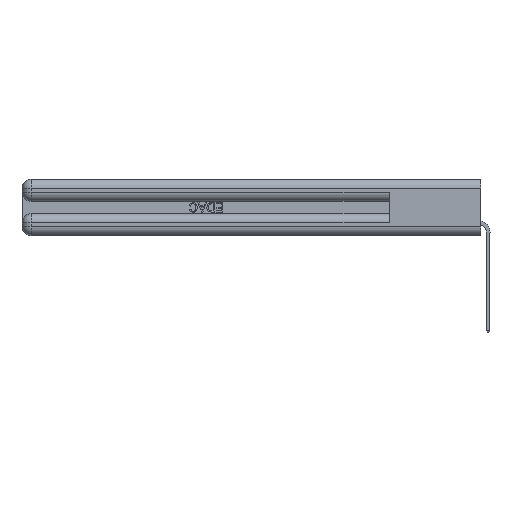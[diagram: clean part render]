
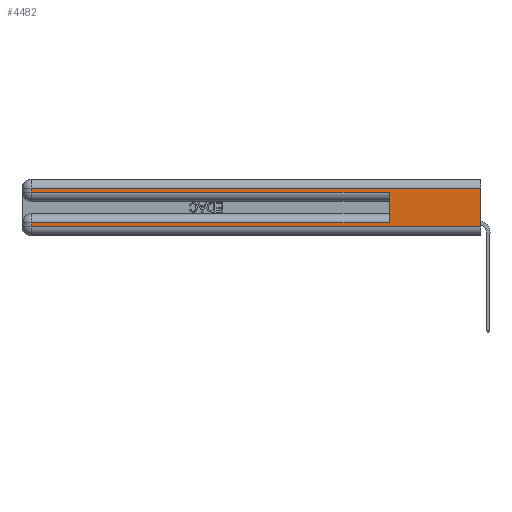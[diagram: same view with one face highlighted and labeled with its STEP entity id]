
A CAD part, left-side view. The second image highlights one B-rep face of the part: STEP entity #4482.
In plain terms, the highlighted planar face has unit normal (-1, 0, 0).
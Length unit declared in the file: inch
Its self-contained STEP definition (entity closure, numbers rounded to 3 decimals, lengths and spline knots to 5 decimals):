
#642 = EDGE_CURVE ( 'NONE', #20522, #5445, #36103, .T. ) ;
#1931 = FACE_OUTER_BOUND ( 'NONE', #25364, .T. ) ;
#2450 = EDGE_CURVE ( 'NONE', #24085, #14892, #4341, .T. ) ;
#4311 = VECTOR ( 'NONE', #20294, 39.37008 ) ;
#4341 = LINE ( 'NONE', #31366, #31011 ) ;
#4423 = ORIENTED_EDGE ( 'NONE', *, *, #25893, .F. ) ;
#4482 = ADVANCED_FACE ( 'NONE', ( #1931 ), #22855, .F. ) ;
#5445 = VERTEX_POINT ( 'NONE', #17617 ) ;
#5885 = DIRECTION ( 'NONE',  ( 1., 0., 0. ) ) ;
#6521 = LINE ( 'NONE', #22173, #24303 ) ;
#6970 = CARTESIAN_POINT ( 'NONE',  ( 0., 2.94, 0.06 ) ) ;
#8982 = ORIENTED_EDGE ( 'NONE', *, *, #10258, .T. ) ;
#9415 = VERTEX_POINT ( 'NONE', #13876 ) ;
#10258 = EDGE_CURVE ( 'NONE', #14892, #24863, #6521, .T. ) ;
#10935 = ORIENTED_EDGE ( 'NONE', *, *, #14495, .T. ) ;
#12194 = VERTEX_POINT ( 'NONE', #35616 ) ;
#13784 = VECTOR ( 'NONE', #21366, 39.37008 ) ;
#13876 = CARTESIAN_POINT ( 'NONE',  ( 0., 2.94, 0.285 ) ) ;
#14004 = CARTESIAN_POINT ( 'NONE',  ( 0., 0., 0.06 ) ) ;
#14495 = EDGE_CURVE ( 'NONE', #24863, #28675, #35197, .T. ) ;
#14892 = VERTEX_POINT ( 'NONE', #22934 ) ;
#15370 = LINE ( 'NONE', #22130, #25187 ) ;
#15599 = DIRECTION ( 'NONE',  ( 0., 0., 1. ) ) ;
#17617 = CARTESIAN_POINT ( 'NONE',  ( 0., 2.94, 0.31 ) ) ;
#18200 = CARTESIAN_POINT ( 'NONE',  ( 0., 0., 0.31 ) ) ;
#19523 = DIRECTION ( 'NONE',  ( 0., 0., -1. ) ) ;
#19554 = VECTOR ( 'NONE', #32605, 39.37008 ) ;
#20106 = CARTESIAN_POINT ( 'NONE',  ( 0., 0., 0.37 ) ) ;
#20294 = DIRECTION ( 'NONE',  ( 0., 0., -1. ) ) ;
#20336 = EDGE_CURVE ( 'NONE', #24085, #12194, #34564, .T. ) ;
#20522 = VERTEX_POINT ( 'NONE', #18200 ) ;
#21243 = CARTESIAN_POINT ( 'NONE',  ( 0., 0., 0.31 ) ) ;
#21366 = DIRECTION ( 'NONE',  ( 0., 1., 0. ) ) ;
#22130 = CARTESIAN_POINT ( 'NONE',  ( 0., 0., 0.37 ) ) ;
#22173 = CARTESIAN_POINT ( 'NONE',  ( 0., 2.94, 0.37 ) ) ;
#22743 = DIRECTION ( 'NONE',  ( 0., 1., 0. ) ) ;
#22776 = ORIENTED_EDGE ( 'NONE', *, *, #27675, .T. ) ;
#22855 = PLANE ( 'NONE',  #29659 ) ;
#22934 = CARTESIAN_POINT ( 'NONE',  ( 0., 2.94, 0.085 ) ) ;
#23114 = DIRECTION ( 'NONE',  ( 0., -1., 0. ) ) ;
#23347 = VECTOR ( 'NONE', #15599, 39.37008 ) ;
#23715 = ORIENTED_EDGE ( 'NONE', *, *, #2450, .T. ) ;
#24085 = VERTEX_POINT ( 'NONE', #28617 ) ;
#24209 = CARTESIAN_POINT ( 'NONE',  ( 0., 0.6, 0.145 ) ) ;
#24223 = ORIENTED_EDGE ( 'NONE', *, *, #642, .T. ) ;
#24303 = VECTOR ( 'NONE', #19523, 39.37008 ) ;
#24863 = VERTEX_POINT ( 'NONE', #6970 ) ;
#25187 = VECTOR ( 'NONE', #30887, 39.37008 ) ;
#25364 = EDGE_LOOP ( 'NONE', ( #4423, #24223, #27951, #22776, #32324, #23715, #8982, #10935 ) ) ;
#25727 = DIRECTION ( 'NONE',  ( 0., 0., -1. ) ) ;
#25893 = EDGE_CURVE ( 'NONE', #20522, #28675, #15370, .T. ) ;
#26285 = CARTESIAN_POINT ( 'NONE',  ( 0., 2.94, 0.37 ) ) ;
#26745 = CARTESIAN_POINT ( 'NONE',  ( 0., 0., 0.06 ) ) ;
#27398 = LINE ( 'NONE', #26285, #4311 ) ;
#27675 = EDGE_CURVE ( 'NONE', #9415, #12194, #32845, .T. ) ;
#27951 = ORIENTED_EDGE ( 'NONE', *, *, #28864, .T. ) ;
#28617 = CARTESIAN_POINT ( 'NONE',  ( 0., 0.6, 0.085 ) ) ;
#28675 = VERTEX_POINT ( 'NONE', #14004 ) ;
#28864 = EDGE_CURVE ( 'NONE', #5445, #9415, #27398, .T. ) ;
#29659 = AXIS2_PLACEMENT_3D ( 'NONE', #20106, #5885, #25727 ) ;
#30887 = DIRECTION ( 'NONE',  ( 0., 0., -1. ) ) ;
#31011 = VECTOR ( 'NONE', #22743, 39.37008 ) ;
#31366 = CARTESIAN_POINT ( 'NONE',  ( 0., 0., 0.085 ) ) ;
#31491 = VECTOR ( 'NONE', #23114, 39.37008 ) ;
#32324 = ORIENTED_EDGE ( 'NONE', *, *, #20336, .F. ) ;
#32605 = DIRECTION ( 'NONE',  ( 0., -1., 0. ) ) ;
#32845 = LINE ( 'NONE', #35130, #31491 ) ;
#34564 = LINE ( 'NONE', #24209, #23347 ) ;
#35130 = CARTESIAN_POINT ( 'NONE',  ( 0., 0., 0.285 ) ) ;
#35197 = LINE ( 'NONE', #26745, #19554 ) ;
#35616 = CARTESIAN_POINT ( 'NONE',  ( 0., 0.6, 0.285 ) ) ;
#36103 = LINE ( 'NONE', #21243, #13784 ) ;
